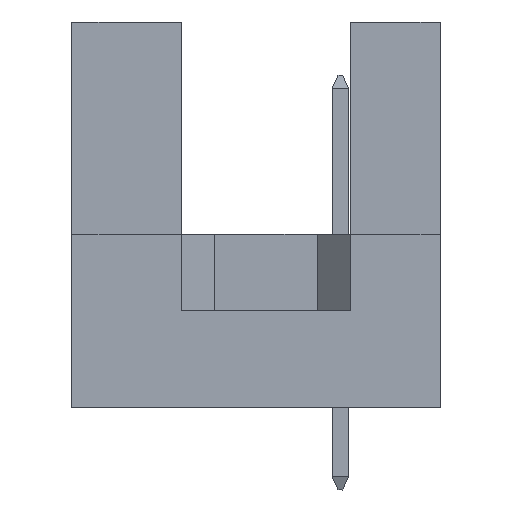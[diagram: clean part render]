
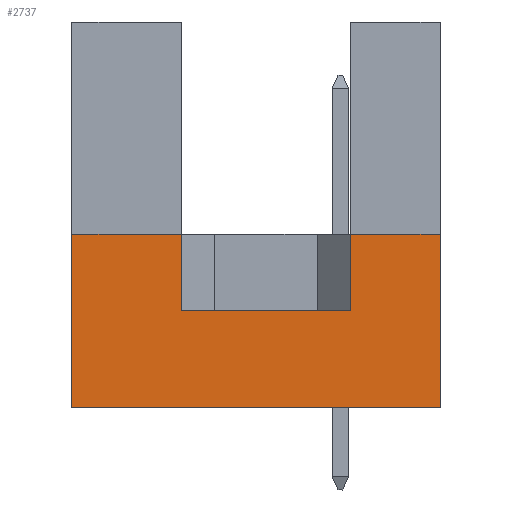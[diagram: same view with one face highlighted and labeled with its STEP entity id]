
A CAD part, left-side view. The second image highlights one B-rep face of the part: STEP entity #2737.
In plain terms, the highlighted planar face has unit normal (-1, 0, 0).
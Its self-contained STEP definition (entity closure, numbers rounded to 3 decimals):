
#185 = CARTESIAN_POINT ( 'NONE',  ( -47.5, 2.71, 5.2 ) ) ;
#428 = EDGE_CURVE ( 'NONE', #2115, #6036, #5259, .T. ) ;
#596 = LINE ( 'NONE', #14139, #13431 ) ;
#783 = CARTESIAN_POINT ( 'NONE',  ( -47.5, 2.71, 2.9 ) ) ;
#826 = DIRECTION ( 'NONE',  ( 0., 0., 1. ) ) ;
#912 = CARTESIAN_POINT ( 'NONE',  ( -47.5, 7.79, 2.9 ) ) ;
#1390 = VECTOR ( 'NONE', #11186, 1000. ) ;
#1513 = CARTESIAN_POINT ( 'NONE',  ( -47.5, 0., 5.2 ) ) ;
#1520 = AXIS2_PLACEMENT_3D ( 'NONE', #10755, #6981, #9471 ) ;
#1530 = ORIENTED_EDGE ( 'NONE', *, *, #4095, .F. ) ;
#1611 = LINE ( 'NONE', #9147, #9730 ) ;
#1743 = CARTESIAN_POINT ( 'NONE',  ( -47.5, 7.79, 2.9 ) ) ;
#1808 = CARTESIAN_POINT ( 'NONE',  ( -47.5, 2.71, 2.9 ) ) ;
#1971 = ORIENTED_EDGE ( 'NONE', *, *, #8891, .F. ) ;
#1982 = CARTESIAN_POINT ( 'NONE',  ( -47.5, 11.1, 0. ) ) ;
#2115 = VERTEX_POINT ( 'NONE', #7745 ) ;
#2397 = CARTESIAN_POINT ( 'NONE',  ( -47.5, 0., 0. ) ) ;
#2640 = DIRECTION ( 'NONE',  ( 0., -1., 0. ) ) ;
#2737 = ADVANCED_FACE ( 'NONE', ( #14532 ), #13159, .F. ) ;
#2800 = DIRECTION ( 'NONE',  ( 0., -1., 0. ) ) ;
#3006 = EDGE_CURVE ( 'NONE', #13647, #13802, #1611, .T. ) ;
#3346 = VECTOR ( 'NONE', #2640, 1000. ) ;
#3835 = CARTESIAN_POINT ( 'NONE',  ( -47.5, 11.1, 5.2 ) ) ;
#4095 = EDGE_CURVE ( 'NONE', #2115, #14361, #11885, .T. ) ;
#4231 = DIRECTION ( 'NONE',  ( 0., 0., 1. ) ) ;
#4311 = EDGE_CURVE ( 'NONE', #6448, #13802, #12591, .T. ) ;
#5259 = LINE ( 'NONE', #1743, #9318 ) ;
#5622 = CARTESIAN_POINT ( 'NONE',  ( -47.5, 11.1, 0. ) ) ;
#6036 = VERTEX_POINT ( 'NONE', #6718 ) ;
#6281 = VECTOR ( 'NONE', #9479, 1000. ) ;
#6448 = VERTEX_POINT ( 'NONE', #2397 ) ;
#6718 = CARTESIAN_POINT ( 'NONE',  ( -47.5, 7.79, 5.2 ) ) ;
#6981 = DIRECTION ( 'NONE',  ( 1., 0., 0. ) ) ;
#7745 = CARTESIAN_POINT ( 'NONE',  ( -47.5, 7.79, 2.9 ) ) ;
#8123 = ORIENTED_EDGE ( 'NONE', *, *, #15220, .F. ) ;
#8208 = DIRECTION ( 'NONE',  ( 0., -1., 0. ) ) ;
#8517 = VECTOR ( 'NONE', #8208, 1000. ) ;
#8595 = ORIENTED_EDGE ( 'NONE', *, *, #3006, .F. ) ;
#8891 = EDGE_CURVE ( 'NONE', #12849, #6036, #11377, .T. ) ;
#9147 = CARTESIAN_POINT ( 'NONE',  ( -47.5, 11.1, 5.2 ) ) ;
#9309 = CARTESIAN_POINT ( 'NONE',  ( -47.5, 0., 0. ) ) ;
#9318 = VECTOR ( 'NONE', #4231, 1000. ) ;
#9471 = DIRECTION ( 'NONE',  ( 0., 0., -1. ) ) ;
#9473 = VERTEX_POINT ( 'NONE', #1982 ) ;
#9479 = DIRECTION ( 'NONE',  ( 0., -1., 0. ) ) ;
#9730 = VECTOR ( 'NONE', #2800, 1000. ) ;
#9967 = ORIENTED_EDGE ( 'NONE', *, *, #428, .T. ) ;
#10338 = CARTESIAN_POINT ( 'NONE',  ( -47.5, 11.1, 5.2 ) ) ;
#10428 = DIRECTION ( 'NONE',  ( 0., 0., 1. ) ) ;
#10755 = CARTESIAN_POINT ( 'NONE',  ( -47.5, 11.1, 0. ) ) ;
#10788 = EDGE_CURVE ( 'NONE', #9473, #6448, #15661, .T. ) ;
#10981 = ORIENTED_EDGE ( 'NONE', *, *, #4311, .T. ) ;
#11186 = DIRECTION ( 'NONE',  ( 0., 0., 1. ) ) ;
#11377 = LINE ( 'NONE', #3835, #3346 ) ;
#11885 = LINE ( 'NONE', #912, #6281 ) ;
#12180 = ORIENTED_EDGE ( 'NONE', *, *, #10788, .T. ) ;
#12591 = LINE ( 'NONE', #9309, #13061 ) ;
#12849 = VERTEX_POINT ( 'NONE', #10338 ) ;
#12965 = ORIENTED_EDGE ( 'NONE', *, *, #14709, .F. ) ;
#13061 = VECTOR ( 'NONE', #10428, 1000. ) ;
#13159 = PLANE ( 'NONE',  #1520 ) ;
#13431 = VECTOR ( 'NONE', #826, 1000. ) ;
#13647 = VERTEX_POINT ( 'NONE', #185 ) ;
#13802 = VERTEX_POINT ( 'NONE', #1513 ) ;
#13911 = LINE ( 'NONE', #1808, #1390 ) ;
#14139 = CARTESIAN_POINT ( 'NONE',  ( -47.5, 11.1, 0. ) ) ;
#14361 = VERTEX_POINT ( 'NONE', #783 ) ;
#14508 = EDGE_LOOP ( 'NONE', ( #1530, #9967, #1971, #8123, #12180, #10981, #8595, #12965 ) ) ;
#14532 = FACE_OUTER_BOUND ( 'NONE', #14508, .T. ) ;
#14709 = EDGE_CURVE ( 'NONE', #14361, #13647, #13911, .T. ) ;
#15220 = EDGE_CURVE ( 'NONE', #9473, #12849, #596, .T. ) ;
#15661 = LINE ( 'NONE', #5622, #8517 ) ;
